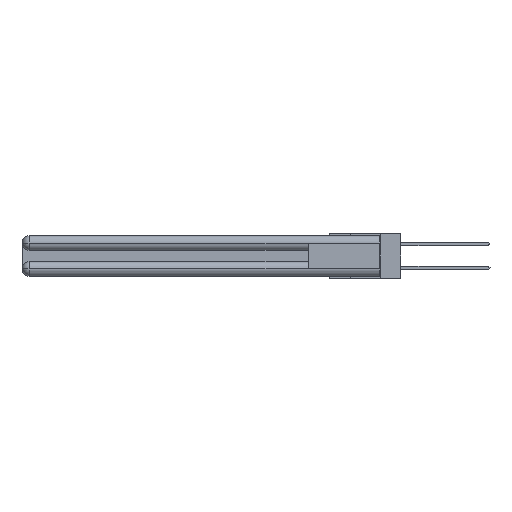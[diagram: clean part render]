
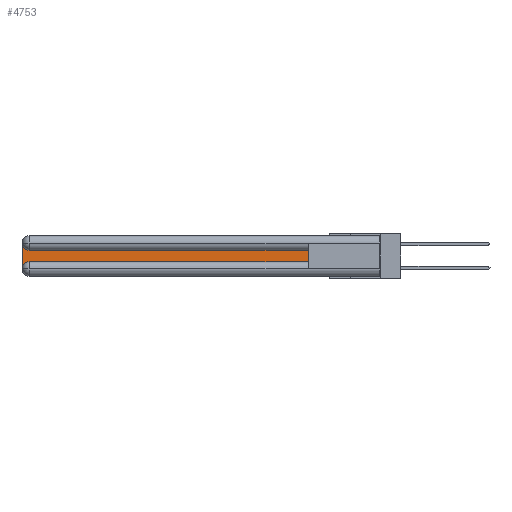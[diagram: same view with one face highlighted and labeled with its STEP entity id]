
A CAD part, left-side view. The second image highlights one B-rep face of the part: STEP entity #4753.
In plain terms, the highlighted planar face has unit normal (-1, 0, 0).
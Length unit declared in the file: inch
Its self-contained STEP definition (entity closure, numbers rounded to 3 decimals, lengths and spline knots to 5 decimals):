
#74 = ORIENTED_EDGE ( 'NONE', *, *, #22075, .T. ) ;
#189 = DIRECTION ( 'NONE',  ( 0., 0., -1. ) ) ;
#297 = CIRCLE ( 'NONE', #17362, 0.06 ) ;
#1754 = CARTESIAN_POINT ( 'NONE',  ( 0.075, 3., -0.2175 ) ) ;
#2100 = CARTESIAN_POINT ( 'NONE',  ( 0.075, 2.94, -0.0625 ) ) ;
#3295 = ORIENTED_EDGE ( 'NONE', *, *, #17279, .T. ) ;
#3577 = VECTOR ( 'NONE', #6685, 39.37008 ) ;
#4242 = LINE ( 'NONE', #1754, #5374 ) ;
#4539 = ORIENTED_EDGE ( 'NONE', *, *, #21025, .T. ) ;
#4753 = ADVANCED_FACE ( 'NONE', ( #18564 ), #8148, .F. ) ;
#5374 = VECTOR ( 'NONE', #11090, 39.37008 ) ;
#5620 = VERTEX_POINT ( 'NONE', #19969 ) ;
#6066 = ORIENTED_EDGE ( 'NONE', *, *, #9481, .T. ) ;
#6263 = AXIS2_PLACEMENT_3D ( 'NONE', #24336, #24700, #29434 ) ;
#6635 = DIRECTION ( 'NONE',  ( 0., 0., -1. ) ) ;
#6685 = DIRECTION ( 'NONE',  ( 0., 1., 0. ) ) ;
#7063 = VECTOR ( 'NONE', #17816, 39.37008 ) ;
#7756 = CARTESIAN_POINT ( 'NONE',  ( 0.075, 0.6, -0.2175 ) ) ;
#8092 = CARTESIAN_POINT ( 'NONE',  ( 0.075, 0.6, -0.2175 ) ) ;
#8148 = PLANE ( 'NONE',  #6263 ) ;
#8846 = EDGE_CURVE ( 'NONE', #17980, #25365, #24284, .T. ) ;
#9035 = CIRCLE ( 'NONE', #15538, 0.06 ) ;
#9481 = EDGE_CURVE ( 'NONE', #26574, #22112, #297, .T. ) ;
#9953 = CARTESIAN_POINT ( 'NONE',  ( 0.075, 3., -0.2775 ) ) ;
#10960 = VERTEX_POINT ( 'NONE', #9953 ) ;
#11090 = DIRECTION ( 'NONE',  ( 0., 0., -1. ) ) ;
#11736 = DIRECTION ( 'NONE',  ( 1., 0., 0. ) ) ;
#13181 = LINE ( 'NONE', #20069, #7063 ) ;
#13356 = CARTESIAN_POINT ( 'NONE',  ( 0.075, 2.94, -0.1225 ) ) ;
#14140 = CARTESIAN_POINT ( 'NONE',  ( 0.075, 2.94, -0.2175 ) ) ;
#15538 = AXIS2_PLACEMENT_3D ( 'NONE', #20668, #23035, #6635 ) ;
#15563 = ORIENTED_EDGE ( 'NONE', *, *, #8846, .T. ) ;
#16039 = ORIENTED_EDGE ( 'NONE', *, *, #23318, .T. ) ;
#17279 = EDGE_CURVE ( 'NONE', #10960, #17980, #9035, .T. ) ;
#17362 = AXIS2_PLACEMENT_3D ( 'NONE', #2100, #11736, #189 ) ;
#17816 = DIRECTION ( 'NONE',  ( 0., 0., 1. ) ) ;
#17980 = VERTEX_POINT ( 'NONE', #14140 ) ;
#18029 = VECTOR ( 'NONE', #20157, 39.37008 ) ;
#18564 = FACE_OUTER_BOUND ( 'NONE', #20581, .T. ) ;
#19969 = CARTESIAN_POINT ( 'NONE',  ( 0.075, 0.6, -0.1225 ) ) ;
#20069 = CARTESIAN_POINT ( 'NONE',  ( 0.075, 0.6, -0.2175 ) ) ;
#20157 = DIRECTION ( 'NONE',  ( 0., -1., 0. ) ) ;
#20581 = EDGE_LOOP ( 'NONE', ( #4539, #6066, #74, #3295, #15563, #16039 ) ) ;
#20668 = CARTESIAN_POINT ( 'NONE',  ( 0.075, 2.94, -0.2775 ) ) ;
#21025 = EDGE_CURVE ( 'NONE', #5620, #26574, #26057, .T. ) ;
#22075 = EDGE_CURVE ( 'NONE', #22112, #10960, #4242, .T. ) ;
#22112 = VERTEX_POINT ( 'NONE', #25146 ) ;
#23035 = DIRECTION ( 'NONE',  ( 1., 0., 0. ) ) ;
#23318 = EDGE_CURVE ( 'NONE', #25365, #5620, #13181, .T. ) ;
#24284 = LINE ( 'NONE', #7756, #18029 ) ;
#24336 = CARTESIAN_POINT ( 'NONE',  ( 0.075, 3., -0.1225 ) ) ;
#24519 = CARTESIAN_POINT ( 'NONE',  ( 0.075, 0.6, -0.1225 ) ) ;
#24700 = DIRECTION ( 'NONE',  ( 1., 0., 0. ) ) ;
#25146 = CARTESIAN_POINT ( 'NONE',  ( 0.075, 3., -0.0625 ) ) ;
#25365 = VERTEX_POINT ( 'NONE', #8092 ) ;
#26057 = LINE ( 'NONE', #24519, #3577 ) ;
#26574 = VERTEX_POINT ( 'NONE', #13356 ) ;
#29434 = DIRECTION ( 'NONE',  ( 0., 0., -1. ) ) ;
